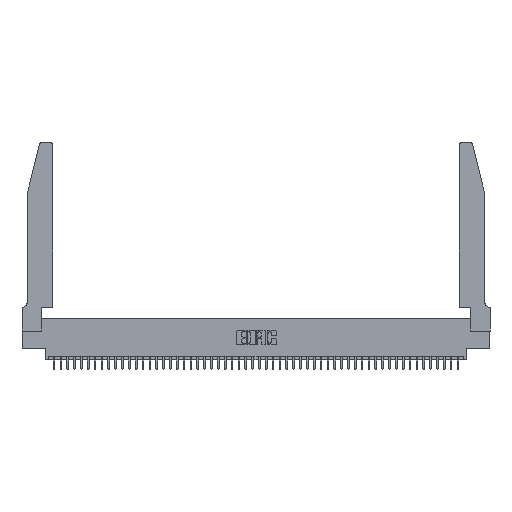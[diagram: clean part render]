
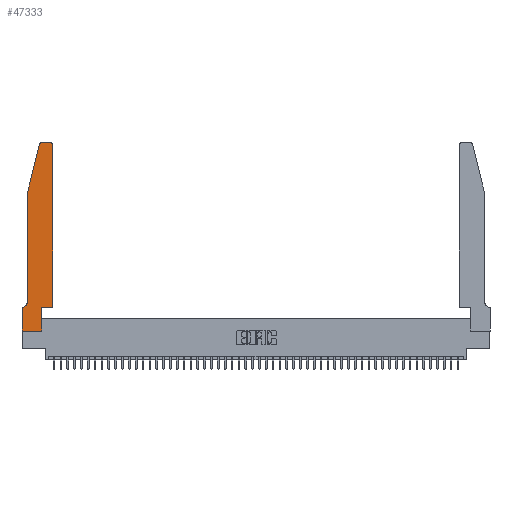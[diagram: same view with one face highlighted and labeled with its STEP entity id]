
A CAD part, top view. The second image highlights one B-rep face of the part: STEP entity #47333.
In plain terms, the highlighted planar face has unit normal (0, 0, 1).
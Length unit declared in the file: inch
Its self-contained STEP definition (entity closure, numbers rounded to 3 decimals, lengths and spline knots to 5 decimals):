
#432 = VERTEX_POINT ( 'NONE', #946 ) ;
#446 = LINE ( 'NONE', #34724, #48982 ) ;
#571 = DIRECTION ( 'NONE',  ( -1., 0., 0. ) ) ;
#764 = EDGE_CURVE ( 'NONE', #36375, #32425, #32144, .T. ) ;
#946 = CARTESIAN_POINT ( 'NONE',  ( 0.0755, 0.42, 0.37 ) ) ;
#1072 = CARTESIAN_POINT ( 'NONE',  ( 0., 0., 0.37 ) ) ;
#1302 = EDGE_LOOP ( 'NONE', ( #4898, #12098, #2145, #25157, #38850, #25493, #4313, #24268, #30984, #24713, #41784, #30533 ) ) ;
#2145 = ORIENTED_EDGE ( 'NONE', *, *, #5224, .T. ) ;
#2196 = DIRECTION ( 'NONE',  ( 0., -1., 0. ) ) ;
#3101 = DIRECTION ( 'NONE',  ( 1., 0., 0. ) ) ;
#3733 = CARTESIAN_POINT ( 'NONE',  ( 0.2865, 0., 0.37 ) ) ;
#4313 = ORIENTED_EDGE ( 'NONE', *, *, #11299, .T. ) ;
#4898 = ORIENTED_EDGE ( 'NONE', *, *, #5093, .T. ) ;
#5093 = EDGE_CURVE ( 'NONE', #39583, #37453, #41210, .T. ) ;
#5159 = CARTESIAN_POINT ( 'NONE',  ( 0.2865, 0.35, 0.37 ) ) ;
#5224 = EDGE_CURVE ( 'NONE', #30640, #48989, #18498, .T. ) ;
#6406 = VECTOR ( 'NONE', #27969, 39.37008 ) ;
#7113 = VECTOR ( 'NONE', #7975, 39.37008 ) ;
#7469 = DIRECTION ( 'NONE',  ( -1., 0., 0. ) ) ;
#7975 = DIRECTION ( 'NONE',  ( -0.239, -0.971, 0. ) ) ;
#8134 = EDGE_CURVE ( 'NONE', #20051, #12073, #11496, .T. ) ;
#8216 = LINE ( 'NONE', #13830, #27379 ) ;
#8835 = VECTOR ( 'NONE', #27555, 39.37008 ) ;
#9368 = VECTOR ( 'NONE', #3101, 39.37008 ) ;
#9648 = CARTESIAN_POINT ( 'NONE',  ( 0.284, 2.75, 0.37 ) ) ;
#10672 = DIRECTION ( 'NONE',  ( -1., 0., 0. ) ) ;
#11117 = DIRECTION ( 'NONE',  ( 0., 0., 1. ) ) ;
#11138 = DIRECTION ( 'NONE',  ( 0., 1., 0. ) ) ;
#11299 = EDGE_CURVE ( 'NONE', #12073, #37464, #39328, .T. ) ;
#11496 = LINE ( 'NONE', #29764, #20487 ) ;
#11566 = EDGE_CURVE ( 'NONE', #48989, #432, #8216, .T. ) ;
#12073 = VERTEX_POINT ( 'NONE', #36997 ) ;
#12098 = ORIENTED_EDGE ( 'NONE', *, *, #44591, .T. ) ;
#13830 = CARTESIAN_POINT ( 'NONE',  ( 0.0755, 2., 0.37 ) ) ;
#15237 = CARTESIAN_POINT ( 'NONE',  ( 0.0755, 2., 0.37 ) ) ;
#15650 = AXIS2_PLACEMENT_3D ( 'NONE', #20644, #47381, #24494 ) ;
#15948 = AXIS2_PLACEMENT_3D ( 'NONE', #34027, #11117, #37865 ) ;
#16024 = AXIS2_PLACEMENT_3D ( 'NONE', #38571, #19522, #46293 ) ;
#17159 = EDGE_CURVE ( 'NONE', #37464, #34991, #35738, .T. ) ;
#17356 = CARTESIAN_POINT ( 'NONE',  ( 0., 0., 0.37 ) ) ;
#17777 = CIRCLE ( 'NONE', #15650, 0.03 ) ;
#18436 = AXIS2_PLACEMENT_3D ( 'NONE', #46496, #23566, #571 ) ;
#18498 = LINE ( 'NONE', #34729, #7113 ) ;
#18848 = CARTESIAN_POINT ( 'NONE',  ( 0.2605, 2.75, 0.37 ) ) ;
#19522 = DIRECTION ( 'NONE',  ( 0., 0., 1. ) ) ;
#20051 = VERTEX_POINT ( 'NONE', #20581 ) ;
#20487 = VECTOR ( 'NONE', #10672, 39.37008 ) ;
#20581 = CARTESIAN_POINT ( 'NONE',  ( 0.0055, 0.35, 0.37 ) ) ;
#20644 = CARTESIAN_POINT ( 'NONE',  ( 0.4205, 2.72, 0.37 ) ) ;
#22304 = CARTESIAN_POINT ( 'NONE',  ( 0.4205, 2.75, 0.37 ) ) ;
#22742 = CARTESIAN_POINT ( 'NONE',  ( 0.4505, 0.35, 0.37 ) ) ;
#23014 = CIRCLE ( 'NONE', #15948, 0.03 ) ;
#23566 = DIRECTION ( 'NONE',  ( 0., 0., -1. ) ) ;
#23678 = CARTESIAN_POINT ( 'NONE',  ( 0., 0., 0.37 ) ) ;
#24268 = ORIENTED_EDGE ( 'NONE', *, *, #17159, .T. ) ;
#24494 = DIRECTION ( 'NONE',  ( 1., 0., 0. ) ) ;
#24713 = ORIENTED_EDGE ( 'NONE', *, *, #764, .T. ) ;
#25157 = ORIENTED_EDGE ( 'NONE', *, *, #11566, .T. ) ;
#25172 = FACE_OUTER_BOUND ( 'NONE', #1302, .T. ) ;
#25493 = ORIENTED_EDGE ( 'NONE', *, *, #8134, .T. ) ;
#26519 = CARTESIAN_POINT ( 'NONE',  ( 0.4505, 2.72, 0.37 ) ) ;
#27379 = VECTOR ( 'NONE', #2196, 39.37008 ) ;
#27540 = CARTESIAN_POINT ( 'NONE',  ( 0.25487, 2.72718, 0.37 ) ) ;
#27555 = DIRECTION ( 'NONE',  ( 0., -1., 0. ) ) ;
#27969 = DIRECTION ( 'NONE',  ( 1., 0., 0. ) ) ;
#27992 = CIRCLE ( 'NONE', #18436, 0.07 ) ;
#29764 = CARTESIAN_POINT ( 'NONE',  ( 0.0755, 0.35, 0.37 ) ) ;
#30533 = ORIENTED_EDGE ( 'NONE', *, *, #33905, .T. ) ;
#30640 = VERTEX_POINT ( 'NONE', #27540 ) ;
#30984 = ORIENTED_EDGE ( 'NONE', *, *, #45932, .T. ) ;
#31098 = VECTOR ( 'NONE', #7469, 39.37008 ) ;
#31801 = VERTEX_POINT ( 'NONE', #26519 ) ;
#32144 = LINE ( 'NONE', #48977, #9368 ) ;
#32425 = VERTEX_POINT ( 'NONE', #22742 ) ;
#33905 = EDGE_CURVE ( 'NONE', #31801, #39583, #17777, .T. ) ;
#34027 = CARTESIAN_POINT ( 'NONE',  ( 0.284, 2.72, 0.37 ) ) ;
#34724 = CARTESIAN_POINT ( 'NONE',  ( 0.4505, 0.35, 0.37 ) ) ;
#34729 = CARTESIAN_POINT ( 'NONE',  ( 0.0755, 2., 0.37 ) ) ;
#34753 = PLANE ( 'NONE',  #16024 ) ;
#34991 = VERTEX_POINT ( 'NONE', #3733 ) ;
#35449 = VECTOR ( 'NONE', #11138, 39.37008 ) ;
#35738 = LINE ( 'NONE', #1072, #6406 ) ;
#36375 = VERTEX_POINT ( 'NONE', #5159 ) ;
#36997 = CARTESIAN_POINT ( 'NONE',  ( 0., 0.35, 0.37 ) ) ;
#37453 = VERTEX_POINT ( 'NONE', #9648 ) ;
#37464 = VERTEX_POINT ( 'NONE', #17356 ) ;
#37851 = LINE ( 'NONE', #41726, #35449 ) ;
#37865 = DIRECTION ( 'NONE',  ( 1., 0., 0. ) ) ;
#38571 = CARTESIAN_POINT ( 'NONE',  ( 0., 0.35, 0.37 ) ) ;
#38850 = ORIENTED_EDGE ( 'NONE', *, *, #41798, .T. ) ;
#39328 = LINE ( 'NONE', #23678, #8835 ) ;
#39583 = VERTEX_POINT ( 'NONE', #22304 ) ;
#40572 = EDGE_CURVE ( 'NONE', #32425, #31801, #446, .T. ) ;
#41210 = LINE ( 'NONE', #18848, #31098 ) ;
#41726 = CARTESIAN_POINT ( 'NONE',  ( 0.2865, 0.35, 0.37 ) ) ;
#41784 = ORIENTED_EDGE ( 'NONE', *, *, #40572, .T. ) ;
#41798 = EDGE_CURVE ( 'NONE', #432, #20051, #27992, .T. ) ;
#44591 = EDGE_CURVE ( 'NONE', #37453, #30640, #23014, .T. ) ;
#45932 = EDGE_CURVE ( 'NONE', #34991, #36375, #37851, .T. ) ;
#46270 = DIRECTION ( 'NONE',  ( 0., 1., 0. ) ) ;
#46293 = DIRECTION ( 'NONE',  ( 1., 0., 0. ) ) ;
#46496 = CARTESIAN_POINT ( 'NONE',  ( 0.0055, 0.42, 0.37 ) ) ;
#47333 = ADVANCED_FACE ( 'NONE', ( #25172 ), #34753, .T. ) ;
#47381 = DIRECTION ( 'NONE',  ( 0., 0., 1. ) ) ;
#48977 = CARTESIAN_POINT ( 'NONE',  ( 0.4505, 0.35, 0.37 ) ) ;
#48982 = VECTOR ( 'NONE', #46270, 39.37008 ) ;
#48989 = VERTEX_POINT ( 'NONE', #15237 ) ;
